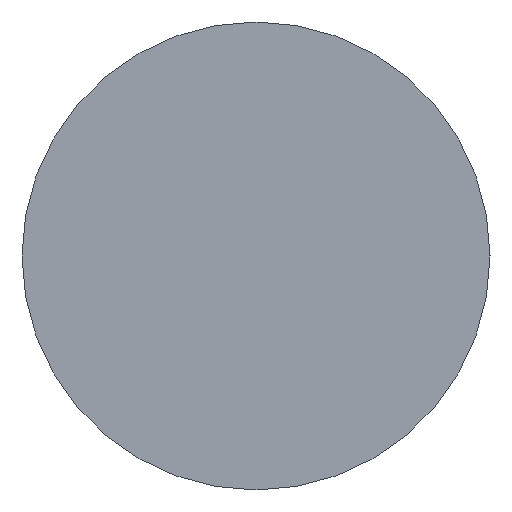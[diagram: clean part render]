
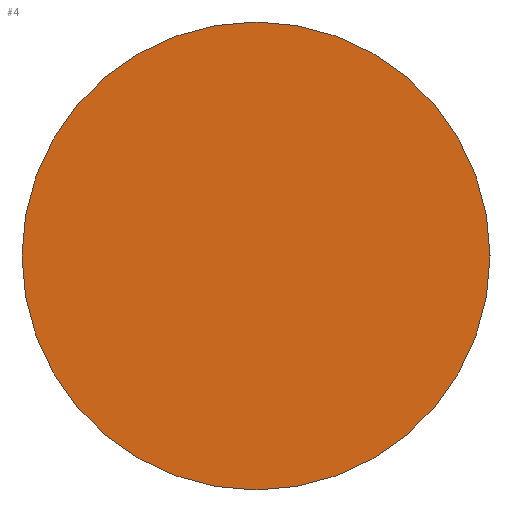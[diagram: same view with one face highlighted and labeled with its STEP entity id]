
A CAD part, left-side view. The second image highlights one B-rep face of the part: STEP entity #4.
In plain terms, the highlighted planar face has unit normal (-1, 0, 0).
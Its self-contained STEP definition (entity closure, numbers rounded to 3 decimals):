
#4 = ADVANCED_FACE ( 'NONE', ( #82 ), #8, .F. ) ;
#8 = PLANE ( 'NONE',  #150 ) ;
#12 = DIRECTION ( 'NONE',  ( 0., 0., -1. ) ) ;
#13 = DIRECTION ( 'NONE',  ( 1., 0., 0. ) ) ;
#14 = CARTESIAN_POINT ( 'NONE',  ( 0., 0., 0. ) ) ;
#24 = CARTESIAN_POINT ( 'NONE',  ( 0., 0., 2. ) ) ;
#51 = DIRECTION ( 'NONE',  ( 0., 0., -1. ) ) ;
#52 = DIRECTION ( 'NONE',  ( 1., 0., 0. ) ) ;
#53 = CARTESIAN_POINT ( 'NONE',  ( 0., 0., 0. ) ) ;
#59 = DIRECTION ( 'NONE',  ( 0., 0., -1. ) ) ;
#60 = DIRECTION ( 'NONE',  ( 1., 0., 0. ) ) ;
#61 = CARTESIAN_POINT ( 'NONE',  ( 0., 0., 0. ) ) ;
#68 = CARTESIAN_POINT ( 'NONE',  ( 0., 0., -2. ) ) ;
#74 = EDGE_LOOP ( 'NONE', ( #91, #92 ) ) ;
#80 = VERTEX_POINT ( 'NONE', #24 ) ;
#82 = FACE_OUTER_BOUND ( 'NONE', #74, .T. ) ;
#83 = VERTEX_POINT ( 'NONE', #68 ) ;
#91 = ORIENTED_EDGE ( 'NONE', *, *, #146, .F. ) ;
#92 = ORIENTED_EDGE ( 'NONE', *, *, #143, .F. ) ;
#96 = CIRCLE ( 'NONE', #151, 2. ) ;
#103 = CIRCLE ( 'NONE', #155, 2. ) ;
#143 = EDGE_CURVE ( 'NONE', #83, #80, #96, .T. ) ;
#146 = EDGE_CURVE ( 'NONE', #80, #83, #103, .T. ) ;
#150 = AXIS2_PLACEMENT_3D ( 'NONE', #14, #13, #12 ) ;
#151 = AXIS2_PLACEMENT_3D ( 'NONE', #61, #60, #59 ) ;
#155 = AXIS2_PLACEMENT_3D ( 'NONE', #53, #52, #51 ) ;
